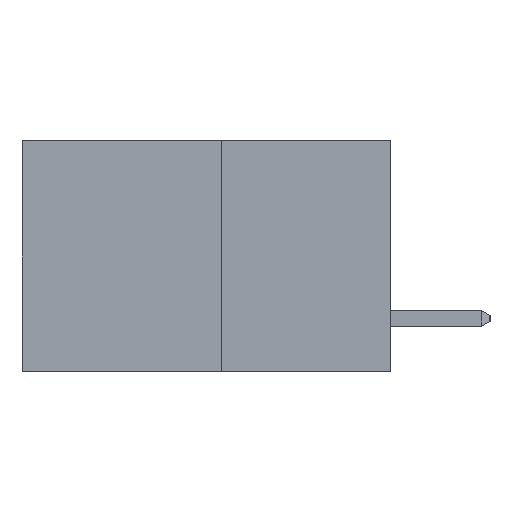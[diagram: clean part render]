
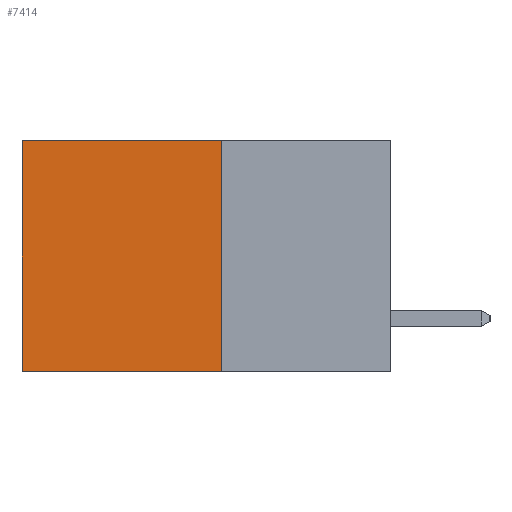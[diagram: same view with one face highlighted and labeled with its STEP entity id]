
A CAD part, left-side view. The second image highlights one B-rep face of the part: STEP entity #7414.
In plain terms, the highlighted planar face has unit normal (-1, 0, 0).
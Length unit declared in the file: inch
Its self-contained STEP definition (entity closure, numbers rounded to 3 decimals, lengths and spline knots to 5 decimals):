
#479 = PLANE ( 'NONE',  #7792 ) ;
#942 = LINE ( 'NONE', #4149, #21272 ) ;
#1763 = LINE ( 'NONE', #17683, #22592 ) ;
#1791 = DIRECTION ( 'NONE',  ( 0., 1., 0. ) ) ;
#1999 = EDGE_CURVE ( 'NONE', #16618, #4271, #942, .T. ) ;
#2584 = DIRECTION ( 'NONE',  ( 0., 0., -1. ) ) ;
#2742 = CARTESIAN_POINT ( 'NONE',  ( 0.277, 0.59, 0. ) ) ;
#3664 = VERTEX_POINT ( 'NONE', #12944 ) ;
#3803 = DIRECTION ( 'NONE',  ( 0., 0., -1. ) ) ;
#4149 = CARTESIAN_POINT ( 'NONE',  ( 0.277, 0.59, -0.37 ) ) ;
#4239 = DIRECTION ( 'NONE',  ( 0., 0., -1. ) ) ;
#4271 = VERTEX_POINT ( 'NONE', #14740 ) ;
#5645 = CARTESIAN_POINT ( 'NONE',  ( 0.277, 0.27, 0. ) ) ;
#7414 = ADVANCED_FACE ( 'NONE', ( #14874 ), #479, .F. ) ;
#7675 = DIRECTION ( 'NONE',  ( 0., 1., 0. ) ) ;
#7792 = AXIS2_PLACEMENT_3D ( 'NONE', #12619, #14642, #2584 ) ;
#7926 = ORIENTED_EDGE ( 'NONE', *, *, #1999, .T. ) ;
#9259 = ORIENTED_EDGE ( 'NONE', *, *, #21921, .T. ) ;
#10809 = EDGE_CURVE ( 'NONE', #3664, #4271, #16581, .T. ) ;
#10835 = ORIENTED_EDGE ( 'NONE', *, *, #13164, .F. ) ;
#11394 = LINE ( 'NONE', #5645, #16059 ) ;
#11830 = CARTESIAN_POINT ( 'NONE',  ( 0.277, 0.27, -0.37 ) ) ;
#12504 = ORIENTED_EDGE ( 'NONE', *, *, #10809, .F. ) ;
#12619 = CARTESIAN_POINT ( 'NONE',  ( 0.277, 0.27, -0.37 ) ) ;
#12944 = CARTESIAN_POINT ( 'NONE',  ( 0.277, 0.27, -0.37 ) ) ;
#13164 = EDGE_CURVE ( 'NONE', #22039, #3664, #1763, .T. ) ;
#14642 = DIRECTION ( 'NONE',  ( 1., 0., 0. ) ) ;
#14740 = CARTESIAN_POINT ( 'NONE',  ( 0.277, 0.59, -0.37 ) ) ;
#14874 = FACE_OUTER_BOUND ( 'NONE', #22171, .T. ) ;
#16001 = VECTOR ( 'NONE', #1791, 39.37008 ) ;
#16059 = VECTOR ( 'NONE', #7675, 39.37008 ) ;
#16581 = LINE ( 'NONE', #11830, #16001 ) ;
#16618 = VERTEX_POINT ( 'NONE', #2742 ) ;
#17683 = CARTESIAN_POINT ( 'NONE',  ( 0.277, 0.27, -0.37 ) ) ;
#19698 = CARTESIAN_POINT ( 'NONE',  ( 0.277, 0.27, 0. ) ) ;
#21272 = VECTOR ( 'NONE', #4239, 39.37008 ) ;
#21921 = EDGE_CURVE ( 'NONE', #22039, #16618, #11394, .T. ) ;
#22039 = VERTEX_POINT ( 'NONE', #19698 ) ;
#22171 = EDGE_LOOP ( 'NONE', ( #7926, #12504, #10835, #9259 ) ) ;
#22592 = VECTOR ( 'NONE', #3803, 39.37008 ) ;
